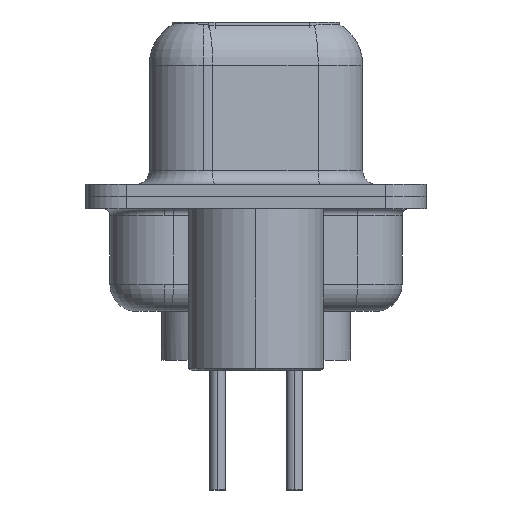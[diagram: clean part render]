
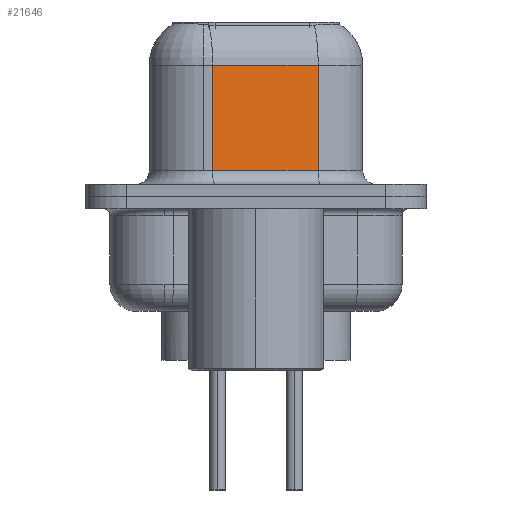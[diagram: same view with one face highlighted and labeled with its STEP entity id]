
A CAD part, left-side view. The second image highlights one B-rep face of the part: STEP entity #21646.
In plain terms, the highlighted planar face has unit normal (-0.985, -0.174, 0).
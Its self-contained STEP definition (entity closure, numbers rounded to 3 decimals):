
#292 = CARTESIAN_POINT ( 'NONE',  ( 5.053, -2.297, 0.95 ) ) ;
#321 = VECTOR ( 'NONE', #19877, 1000. ) ;
#935 = ORIENTED_EDGE ( 'NONE', *, *, #4969, .F. ) ;
#2421 = EDGE_CURVE ( 'NONE', #9075, #16406, #16099, .T. ) ;
#2913 = AXIS2_PLACEMENT_3D ( 'NONE', #6090, #11359, #18720 ) ;
#4130 = ORIENTED_EDGE ( 'NONE', *, *, #2421, .T. ) ;
#4290 = CARTESIAN_POINT ( 'NONE',  ( 5.053, -2.297, 4.85 ) ) ;
#4790 = EDGE_CURVE ( 'NONE', #21978, #9075, #8669, .T. ) ;
#4815 = EDGE_CURVE ( 'NONE', #16406, #16788, #15843, .T. ) ;
#4855 = CARTESIAN_POINT ( 'NONE',  ( 4.365, 1.603, 0.95 ) ) ;
#4969 = EDGE_CURVE ( 'NONE', #21978, #16788, #8853, .T. ) ;
#6090 = CARTESIAN_POINT ( 'NONE',  ( 5.053, -2.297, 6.6 ) ) ;
#6790 = EDGE_LOOP ( 'NONE', ( #935, #11364, #4130, #19556 ) ) ;
#8064 = PLANE ( 'NONE',  #2913 ) ;
#8669 = LINE ( 'NONE', #9257, #9923 ) ;
#8853 = LINE ( 'NONE', #23982, #19883 ) ;
#9075 = VERTEX_POINT ( 'NONE', #17854 ) ;
#9257 = CARTESIAN_POINT ( 'NONE',  ( 5.053, -2.297, 4.85 ) ) ;
#9923 = VECTOR ( 'NONE', #23917, 1000. ) ;
#11359 = DIRECTION ( 'NONE',  ( 0.985, 0.174, 0. ) ) ;
#11364 = ORIENTED_EDGE ( 'NONE', *, *, #4790, .T. ) ;
#15843 = LINE ( 'NONE', #292, #18282 ) ;
#16099 = LINE ( 'NONE', #16350, #321 ) ;
#16350 = CARTESIAN_POINT ( 'NONE',  ( 4.365, 1.603, 6.6 ) ) ;
#16406 = VERTEX_POINT ( 'NONE', #4855 ) ;
#16788 = VERTEX_POINT ( 'NONE', #23015 ) ;
#17854 = CARTESIAN_POINT ( 'NONE',  ( 4.365, 1.603, 4.85 ) ) ;
#18282 = VECTOR ( 'NONE', #19620, 1000. ) ;
#18720 = DIRECTION ( 'NONE',  ( -0.174, 0.985, 0. ) ) ;
#19556 = ORIENTED_EDGE ( 'NONE', *, *, #4815, .T. ) ;
#19620 = DIRECTION ( 'NONE',  ( 0.174, -0.985, 0. ) ) ;
#19863 = DIRECTION ( 'NONE',  ( 0., 0., -1. ) ) ;
#19877 = DIRECTION ( 'NONE',  ( 0., 0., -1. ) ) ;
#19883 = VECTOR ( 'NONE', #19863, 1000. ) ;
#20835 = FACE_OUTER_BOUND ( 'NONE', #6790, .T. ) ;
#21646 = ADVANCED_FACE ( 'NONE', ( #20835 ), #8064, .F. ) ;
#21978 = VERTEX_POINT ( 'NONE', #4290 ) ;
#23015 = CARTESIAN_POINT ( 'NONE',  ( 5.053, -2.297, 0.95 ) ) ;
#23917 = DIRECTION ( 'NONE',  ( -0.174, 0.985, 0. ) ) ;
#23982 = CARTESIAN_POINT ( 'NONE',  ( 5.053, -2.297, 6.6 ) ) ;
